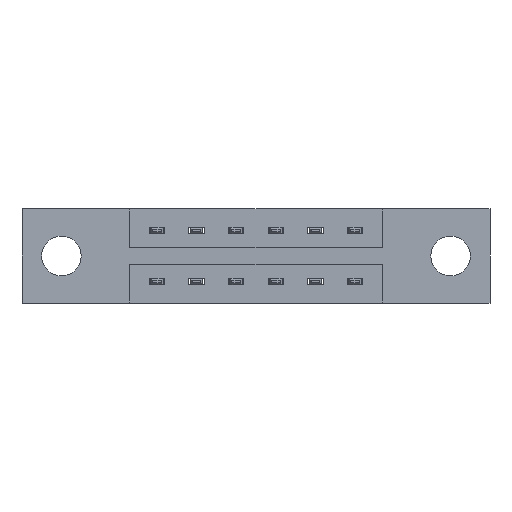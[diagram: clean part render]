
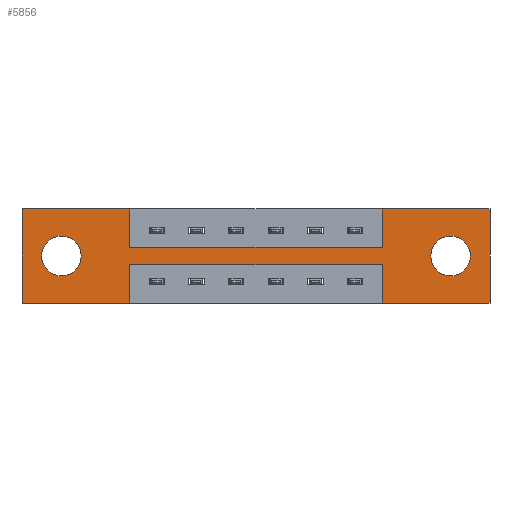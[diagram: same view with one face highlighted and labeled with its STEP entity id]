
A CAD part, front view. The second image highlights one B-rep face of the part: STEP entity #5856.
In plain terms, the highlighted planar face has unit normal (0, -1, 0).
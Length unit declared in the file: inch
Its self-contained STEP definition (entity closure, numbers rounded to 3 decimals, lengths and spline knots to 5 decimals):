
#7 = CARTESIAN_POINT ( 'NONE',  ( 1.687, 0., -0.185 ) ) ;
#31 = VECTOR ( 'NONE', #2128, 39.37008 ) ;
#36 = LINE ( 'NONE', #8972, #2020 ) ;
#89 = DIRECTION ( 'NONE',  ( 0., 0., -1. ) ) ;
#112 = VERTEX_POINT ( 'NONE', #7240 ) ;
#229 = ORIENTED_EDGE ( 'NONE', *, *, #1047, .F. ) ;
#263 = CARTESIAN_POINT ( 'NONE',  ( 1.417, 0., -0.15 ) ) ;
#291 = CARTESIAN_POINT ( 'NONE',  ( 1.417, 0., -0.37 ) ) ;
#327 = DIRECTION ( 'NONE',  ( 0., 0., 1. ) ) ;
#401 = CARTESIAN_POINT ( 'NONE',  ( 0., 0., -0.37 ) ) ;
#405 = VECTOR ( 'NONE', #1136, 39.37008 ) ;
#516 = CARTESIAN_POINT ( 'NONE',  ( 0.425, 0., -0.37 ) ) ;
#638 = EDGE_CURVE ( 'NONE', #112, #9116, #7237, .T. ) ;
#689 = EDGE_CURVE ( 'NONE', #1203, #3691, #4363, .T. ) ;
#826 = EDGE_CURVE ( 'NONE', #4418, #6509, #2377, .T. ) ;
#847 = CIRCLE ( 'NONE', #3101, 0.078 ) ;
#926 = AXIS2_PLACEMENT_3D ( 'NONE', #401, #1812, #1120 ) ;
#927 = ORIENTED_EDGE ( 'NONE', *, *, #689, .F. ) ;
#1047 = EDGE_CURVE ( 'NONE', #2657, #2811, #7905, .T. ) ;
#1053 = FACE_BOUND ( 'NONE', #8506, .T. ) ;
#1118 = CARTESIAN_POINT ( 'NONE',  ( 0.425, 0., -0.22 ) ) ;
#1120 = DIRECTION ( 'NONE',  ( 0., 0., -1. ) ) ;
#1136 = DIRECTION ( 'NONE',  ( 0., 0., -1. ) ) ;
#1145 = VERTEX_POINT ( 'NONE', #3760 ) ;
#1203 = VERTEX_POINT ( 'NONE', #4018 ) ;
#1234 = EDGE_CURVE ( 'NONE', #8157, #4140, #5251, .T. ) ;
#1248 = DIRECTION ( 'NONE',  ( 1., 0., 0. ) ) ;
#1268 = ORIENTED_EDGE ( 'NONE', *, *, #4091, .F. ) ;
#1364 = EDGE_CURVE ( 'NONE', #9116, #4815, #36, .T. ) ;
#1539 = VECTOR ( 'NONE', #89, 39.37008 ) ;
#1580 = VECTOR ( 'NONE', #8259, 39.37008 ) ;
#1740 = DIRECTION ( 'NONE',  ( 0., 1., 0. ) ) ;
#1751 = VECTOR ( 'NONE', #1941, 39.37008 ) ;
#1770 = EDGE_CURVE ( 'NONE', #1816, #8228, #6339, .T. ) ;
#1812 = DIRECTION ( 'NONE',  ( 0., -1., 0. ) ) ;
#1816 = VERTEX_POINT ( 'NONE', #7971 ) ;
#1918 = ORIENTED_EDGE ( 'NONE', *, *, #7470, .F. ) ;
#1919 = VECTOR ( 'NONE', #2734, 39.37008 ) ;
#1941 = DIRECTION ( 'NONE',  ( 0., 0., 1. ) ) ;
#1970 = CARTESIAN_POINT ( 'NONE',  ( 1.417, 0., 0. ) ) ;
#2020 = VECTOR ( 'NONE', #1248, 39.37008 ) ;
#2128 = DIRECTION ( 'NONE',  ( -1., 0., 0. ) ) ;
#2132 = DIRECTION ( 'NONE',  ( 0., 1., 0. ) ) ;
#2168 = VERTEX_POINT ( 'NONE', #8313 ) ;
#2220 = EDGE_LOOP ( 'NONE', ( #1268, #927, #3810, #6994, #7544, #7303, #7585, #229, #4945, #8346, #2584, #1918 ) ) ;
#2268 = LINE ( 'NONE', #7526, #405 ) ;
#2377 = CIRCLE ( 'NONE', #3487, 0.078 ) ;
#2491 = VECTOR ( 'NONE', #9102, 39.37008 ) ;
#2584 = ORIENTED_EDGE ( 'NONE', *, *, #638, .F. ) ;
#2613 = EDGE_CURVE ( 'NONE', #1145, #4509, #4545, .T. ) ;
#2657 = VERTEX_POINT ( 'NONE', #5821 ) ;
#2734 = DIRECTION ( 'NONE',  ( 0., 0., 1. ) ) ;
#2811 = VERTEX_POINT ( 'NONE', #263 ) ;
#2903 = DIRECTION ( 'NONE',  ( 0., 1., 0. ) ) ;
#2993 = CARTESIAN_POINT ( 'NONE',  ( 1.417, 0., -0.37 ) ) ;
#3101 = AXIS2_PLACEMENT_3D ( 'NONE', #7, #2132, #7727 ) ;
#3145 = LINE ( 'NONE', #1970, #1751 ) ;
#3413 = LINE ( 'NONE', #8574, #1539 ) ;
#3436 = DIRECTION ( 'NONE',  ( 0., 0., -1. ) ) ;
#3443 = EDGE_CURVE ( 'NONE', #8228, #1203, #7294, .T. ) ;
#3487 = AXIS2_PLACEMENT_3D ( 'NONE', #8621, #7827, #4288 ) ;
#3493 = CARTESIAN_POINT ( 'NONE',  ( 0., 0., -0.37 ) ) ;
#3595 = EDGE_CURVE ( 'NONE', #4140, #1816, #3413, .T. ) ;
#3668 = CARTESIAN_POINT ( 'NONE',  ( 1.687, 0., -0.185 ) ) ;
#3676 = CARTESIAN_POINT ( 'NONE',  ( 0., 0., 0. ) ) ;
#3691 = VERTEX_POINT ( 'NONE', #1118 ) ;
#3760 = CARTESIAN_POINT ( 'NONE',  ( 1.687, 0., -0.107 ) ) ;
#3810 = ORIENTED_EDGE ( 'NONE', *, *, #3443, .F. ) ;
#3866 = VECTOR ( 'NONE', #8668, 39.37008 ) ;
#4001 = AXIS2_PLACEMENT_3D ( 'NONE', #3668, #2903, #5684 ) ;
#4018 = CARTESIAN_POINT ( 'NONE',  ( 1.417, 0., -0.22 ) ) ;
#4091 = EDGE_CURVE ( 'NONE', #3691, #2168, #6517, .T. ) ;
#4105 = CARTESIAN_POINT ( 'NONE',  ( 0., 0., 0. ) ) ;
#4140 = VERTEX_POINT ( 'NONE', #7156 ) ;
#4288 = DIRECTION ( 'NONE',  ( 0., 0., 1. ) ) ;
#4345 = CARTESIAN_POINT ( 'NONE',  ( 0., 0., 0. ) ) ;
#4363 = LINE ( 'NONE', #5574, #2491 ) ;
#4370 = ORIENTED_EDGE ( 'NONE', *, *, #2613, .T. ) ;
#4372 = CARTESIAN_POINT ( 'NONE',  ( 0.155, 0., -0.263 ) ) ;
#4418 = VERTEX_POINT ( 'NONE', #4372 ) ;
#4509 = VERTEX_POINT ( 'NONE', #4999 ) ;
#4545 = CIRCLE ( 'NONE', #4001, 0.078 ) ;
#4815 = VERTEX_POINT ( 'NONE', #6891 ) ;
#4818 = CARTESIAN_POINT ( 'NONE',  ( 0.155, 0., -0.107 ) ) ;
#4834 = EDGE_CURVE ( 'NONE', #2811, #8157, #3145, .T. ) ;
#4945 = ORIENTED_EDGE ( 'NONE', *, *, #6419, .F. ) ;
#4969 = DIRECTION ( 'NONE',  ( 1., 0., 0. ) ) ;
#4999 = CARTESIAN_POINT ( 'NONE',  ( 1.687, 0., -0.263 ) ) ;
#5011 = VECTOR ( 'NONE', #4969, 39.37008 ) ;
#5143 = DIRECTION ( 'NONE',  ( -1., 0., 0. ) ) ;
#5251 = LINE ( 'NONE', #3676, #5011 ) ;
#5409 = EDGE_CURVE ( 'NONE', #4509, #1145, #847, .T. ) ;
#5478 = CIRCLE ( 'NONE', #8768, 0.078 ) ;
#5574 = CARTESIAN_POINT ( 'NONE',  ( 0.425, 0., -0.22 ) ) ;
#5684 = DIRECTION ( 'NONE',  ( 0., 0., -1. ) ) ;
#5821 = CARTESIAN_POINT ( 'NONE',  ( 0.425, 0., -0.15 ) ) ;
#5856 = ADVANCED_FACE ( 'NONE', ( #7151, #1053, #7258 ), #8955, .T. ) ;
#6003 = CARTESIAN_POINT ( 'NONE',  ( 0.425, 0., -0.15 ) ) ;
#6006 = VECTOR ( 'NONE', #5143, 39.37008 ) ;
#6053 = CARTESIAN_POINT ( 'NONE',  ( 0.155, 0., -0.185 ) ) ;
#6206 = EDGE_CURVE ( 'NONE', #6509, #4418, #5478, .T. ) ;
#6339 = LINE ( 'NONE', #6360, #31 ) ;
#6360 = CARTESIAN_POINT ( 'NONE',  ( 0., 0., -0.37 ) ) ;
#6419 = EDGE_CURVE ( 'NONE', #4815, #2657, #2268, .T. ) ;
#6476 = ORIENTED_EDGE ( 'NONE', *, *, #826, .T. ) ;
#6509 = VERTEX_POINT ( 'NONE', #4818 ) ;
#6517 = LINE ( 'NONE', #516, #7964 ) ;
#6582 = CARTESIAN_POINT ( 'NONE',  ( 1.417, 0., 0. ) ) ;
#6891 = CARTESIAN_POINT ( 'NONE',  ( 0.425, 0., 0. ) ) ;
#6994 = ORIENTED_EDGE ( 'NONE', *, *, #1770, .F. ) ;
#7151 = FACE_BOUND ( 'NONE', #8906, .T. ) ;
#7156 = CARTESIAN_POINT ( 'NONE',  ( 1.842, 0., 0. ) ) ;
#7237 = LINE ( 'NONE', #4105, #1919 ) ;
#7240 = CARTESIAN_POINT ( 'NONE',  ( 0., 0., -0.37 ) ) ;
#7258 = FACE_OUTER_BOUND ( 'NONE', #2220, .T. ) ;
#7294 = LINE ( 'NONE', #2993, #3866 ) ;
#7303 = ORIENTED_EDGE ( 'NONE', *, *, #1234, .F. ) ;
#7470 = EDGE_CURVE ( 'NONE', #2168, #112, #8521, .T. ) ;
#7526 = CARTESIAN_POINT ( 'NONE',  ( 0.425, 0., 0. ) ) ;
#7544 = ORIENTED_EDGE ( 'NONE', *, *, #3595, .F. ) ;
#7585 = ORIENTED_EDGE ( 'NONE', *, *, #4834, .F. ) ;
#7723 = ORIENTED_EDGE ( 'NONE', *, *, #5409, .T. ) ;
#7727 = DIRECTION ( 'NONE',  ( 0., 0., -1. ) ) ;
#7741 = ORIENTED_EDGE ( 'NONE', *, *, #6206, .T. ) ;
#7827 = DIRECTION ( 'NONE',  ( 0., 1., 0. ) ) ;
#7905 = LINE ( 'NONE', #6003, #1580 ) ;
#7964 = VECTOR ( 'NONE', #3436, 39.37008 ) ;
#7971 = CARTESIAN_POINT ( 'NONE',  ( 1.842, 0., -0.37 ) ) ;
#8157 = VERTEX_POINT ( 'NONE', #6582 ) ;
#8228 = VERTEX_POINT ( 'NONE', #291 ) ;
#8259 = DIRECTION ( 'NONE',  ( 1., 0., 0. ) ) ;
#8313 = CARTESIAN_POINT ( 'NONE',  ( 0.425, 0., -0.37 ) ) ;
#8346 = ORIENTED_EDGE ( 'NONE', *, *, #1364, .F. ) ;
#8506 = EDGE_LOOP ( 'NONE', ( #7741, #6476 ) ) ;
#8521 = LINE ( 'NONE', #3493, #6006 ) ;
#8574 = CARTESIAN_POINT ( 'NONE',  ( 1.842, 0., 0. ) ) ;
#8621 = CARTESIAN_POINT ( 'NONE',  ( 0.155, 0., -0.185 ) ) ;
#8668 = DIRECTION ( 'NONE',  ( 0., 0., 1. ) ) ;
#8768 = AXIS2_PLACEMENT_3D ( 'NONE', #6053, #1740, #327 ) ;
#8906 = EDGE_LOOP ( 'NONE', ( #4370, #7723 ) ) ;
#8955 = PLANE ( 'NONE',  #926 ) ;
#8972 = CARTESIAN_POINT ( 'NONE',  ( 0., 0., 0. ) ) ;
#9102 = DIRECTION ( 'NONE',  ( -1., 0., 0. ) ) ;
#9116 = VERTEX_POINT ( 'NONE', #4345 ) ;
